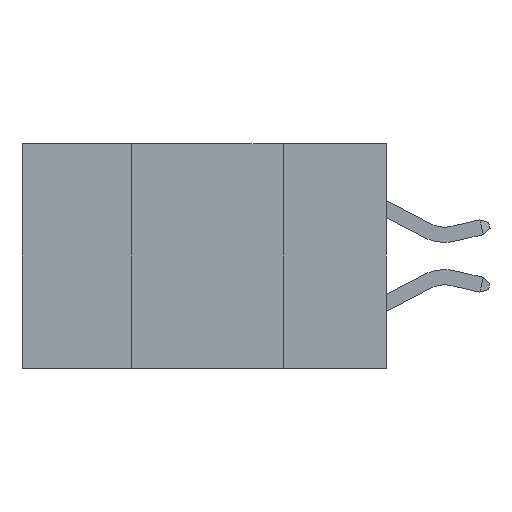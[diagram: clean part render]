
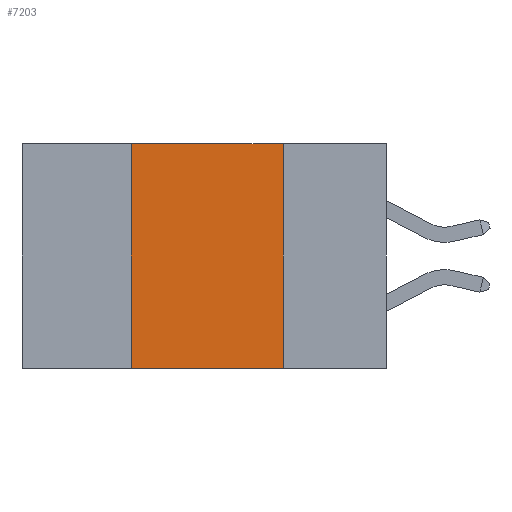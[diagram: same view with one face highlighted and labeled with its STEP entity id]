
A CAD part, left-side view. The second image highlights one B-rep face of the part: STEP entity #7203.
In plain terms, the highlighted planar face has unit normal (-1, 0, 0).
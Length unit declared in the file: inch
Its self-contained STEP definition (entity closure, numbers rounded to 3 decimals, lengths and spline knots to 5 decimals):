
#100 = VERTEX_POINT ( 'NONE', #2770 ) ;
#682 = LINE ( 'NONE', #3687, #7777 ) ;
#849 = VERTEX_POINT ( 'NONE', #7630 ) ;
#1057 = DIRECTION ( 'NONE',  ( 0., -1., 0. ) ) ;
#1073 = CARTESIAN_POINT ( 'NONE',  ( 0., 0.6, -0.37 ) ) ;
#1491 = EDGE_LOOP ( 'NONE', ( #10413, #16621, #6560, #8220 ) ) ;
#2733 = DIRECTION ( 'NONE',  ( 0., -1., 0. ) ) ;
#2770 = CARTESIAN_POINT ( 'NONE',  ( 0., 0.42, -0.37 ) ) ;
#3094 = CARTESIAN_POINT ( 'NONE',  ( 0., 0.17, -0.37 ) ) ;
#3590 = CARTESIAN_POINT ( 'NONE',  ( 0., 0.17, 0. ) ) ;
#3687 = CARTESIAN_POINT ( 'NONE',  ( 0., 0.42, 0. ) ) ;
#4128 = DIRECTION ( 'NONE',  ( 0., 0., -1. ) ) ;
#4373 = EDGE_CURVE ( 'NONE', #100, #4793, #8237, .T. ) ;
#4707 = AXIS2_PLACEMENT_3D ( 'NONE', #13933, #13831, #13668 ) ;
#4793 = VERTEX_POINT ( 'NONE', #3094 ) ;
#5305 = EDGE_CURVE ( 'NONE', #100, #17386, #682, .T. ) ;
#6260 = EDGE_CURVE ( 'NONE', #849, #4793, #12531, .T. ) ;
#6560 = ORIENTED_EDGE ( 'NONE', *, *, #5305, .F. ) ;
#6650 = DIRECTION ( 'NONE',  ( 0., 0., 1. ) ) ;
#7203 = ADVANCED_FACE ( 'NONE', ( #8348 ), #14197, .F. ) ;
#7630 = CARTESIAN_POINT ( 'NONE',  ( 0., 0.17, 0. ) ) ;
#7777 = VECTOR ( 'NONE', #6650, 39.37008 ) ;
#8220 = ORIENTED_EDGE ( 'NONE', *, *, #4373, .T. ) ;
#8237 = LINE ( 'NONE', #1073, #15707 ) ;
#8348 = FACE_OUTER_BOUND ( 'NONE', #1491, .T. ) ;
#10413 = ORIENTED_EDGE ( 'NONE', *, *, #6260, .F. ) ;
#10772 = VECTOR ( 'NONE', #2733, 39.37008 ) ;
#12531 = LINE ( 'NONE', #3590, #15837 ) ;
#12546 = CARTESIAN_POINT ( 'NONE',  ( 0., 0.6, 0. ) ) ;
#13668 = DIRECTION ( 'NONE',  ( 0., 0., -1. ) ) ;
#13716 = LINE ( 'NONE', #12546, #10772 ) ;
#13831 = DIRECTION ( 'NONE',  ( 1., 0., 0. ) ) ;
#13933 = CARTESIAN_POINT ( 'NONE',  ( 0., 0.6, 0. ) ) ;
#14197 = PLANE ( 'NONE',  #4707 ) ;
#15707 = VECTOR ( 'NONE', #1057, 39.37008 ) ;
#15837 = VECTOR ( 'NONE', #4128, 39.37008 ) ;
#16060 = CARTESIAN_POINT ( 'NONE',  ( 0., 0.42, 0. ) ) ;
#16621 = ORIENTED_EDGE ( 'NONE', *, *, #18036, .F. ) ;
#17386 = VERTEX_POINT ( 'NONE', #16060 ) ;
#18036 = EDGE_CURVE ( 'NONE', #17386, #849, #13716, .T. ) ;
